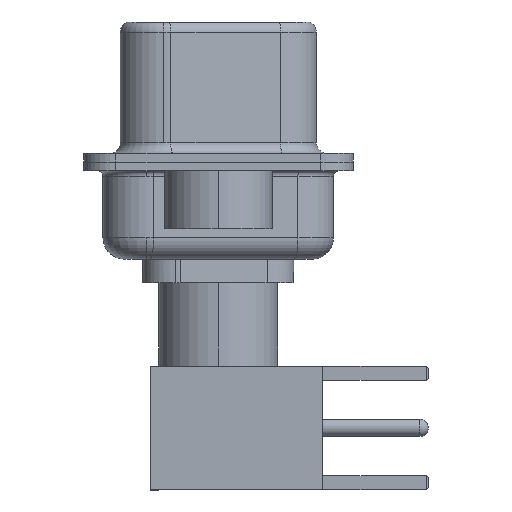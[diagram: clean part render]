
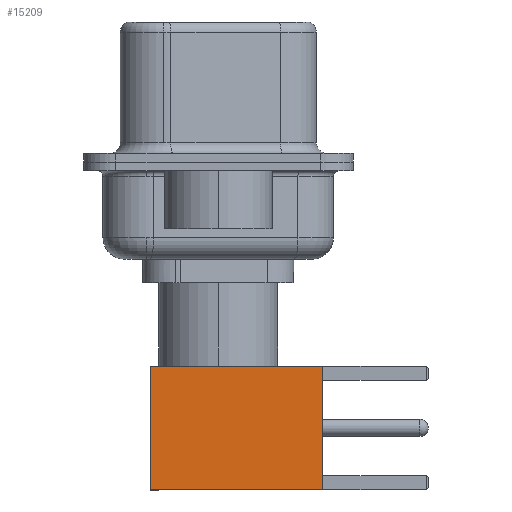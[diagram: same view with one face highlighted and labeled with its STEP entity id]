
A CAD part, left-side view. The second image highlights one B-rep face of the part: STEP entity #15209.
In plain terms, the highlighted face is planar.
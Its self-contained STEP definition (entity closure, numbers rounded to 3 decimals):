
#23 = VECTOR ( 'NONE', #13831, 1000. ) ;
#59 = EDGE_CURVE ( 'NONE', #15554, #2423, #10340, .T. ) ;
#1072 = PLANE ( 'NONE',  #13202 ) ;
#1305 = VECTOR ( 'NONE', #15290, 1000. ) ;
#1545 = CARTESIAN_POINT ( 'NONE',  ( -2.875, 2.875, 0. ) ) ;
#2183 = VERTEX_POINT ( 'NONE', #5858 ) ;
#2423 = VERTEX_POINT ( 'NONE', #8594 ) ;
#2811 = CARTESIAN_POINT ( 'NONE',  ( -2.875, 2.875, 8. ) ) ;
#3396 = CARTESIAN_POINT ( 'NONE',  ( 2.875, 2.875, 0. ) ) ;
#3459 = DIRECTION ( 'NONE',  ( -1., 0., 0. ) ) ;
#5369 = VECTOR ( 'NONE', #3459, 1000. ) ;
#5858 = CARTESIAN_POINT ( 'NONE',  ( 2.875, 2.875, 8. ) ) ;
#6569 = EDGE_LOOP ( 'NONE', ( #10447, #10241, #7727, #7284 ) ) ;
#7081 = FACE_OUTER_BOUND ( 'NONE', #6569, .T. ) ;
#7284 = ORIENTED_EDGE ( 'NONE', *, *, #10625, .F. ) ;
#7490 = LINE ( 'NONE', #1545, #23 ) ;
#7727 = ORIENTED_EDGE ( 'NONE', *, *, #10952, .F. ) ;
#7856 = CARTESIAN_POINT ( 'NONE',  ( 2.875, 2.875, 0. ) ) ;
#7972 = CARTESIAN_POINT ( 'NONE',  ( 2.875, 2.875, 0. ) ) ;
#8135 = CARTESIAN_POINT ( 'NONE',  ( 0., 2.875, 8. ) ) ;
#8594 = CARTESIAN_POINT ( 'NONE',  ( -2.875, 2.875, 0. ) ) ;
#8958 = VERTEX_POINT ( 'NONE', #2811 ) ;
#8967 = EDGE_CURVE ( 'NONE', #2183, #15554, #9145, .T. ) ;
#9145 = LINE ( 'NONE', #7856, #10953 ) ;
#10241 = ORIENTED_EDGE ( 'NONE', *, *, #59, .T. ) ;
#10340 = LINE ( 'NONE', #10778, #5369 ) ;
#10447 = ORIENTED_EDGE ( 'NONE', *, *, #8967, .T. ) ;
#10625 = EDGE_CURVE ( 'NONE', #2183, #8958, #10628, .T. ) ;
#10628 = LINE ( 'NONE', #8135, #1305 ) ;
#10778 = CARTESIAN_POINT ( 'NONE',  ( 0., 2.875, 0. ) ) ;
#10952 = EDGE_CURVE ( 'NONE', #8958, #2423, #7490, .T. ) ;
#10953 = VECTOR ( 'NONE', #11393, 1000. ) ;
#11393 = DIRECTION ( 'NONE',  ( 0., 0., -1. ) ) ;
#13030 = DIRECTION ( 'NONE',  ( 0., 1., 0. ) ) ;
#13202 = AXIS2_PLACEMENT_3D ( 'NONE', #3396, #13030, #13266 ) ;
#13266 = DIRECTION ( 'NONE',  ( 0., 0., 1. ) ) ;
#13831 = DIRECTION ( 'NONE',  ( 0., 0., -1. ) ) ;
#15209 = ADVANCED_FACE ( 'NONE', ( #7081 ), #1072, .T. ) ;
#15290 = DIRECTION ( 'NONE',  ( -1., 0., 0. ) ) ;
#15554 = VERTEX_POINT ( 'NONE', #7972 ) ;
